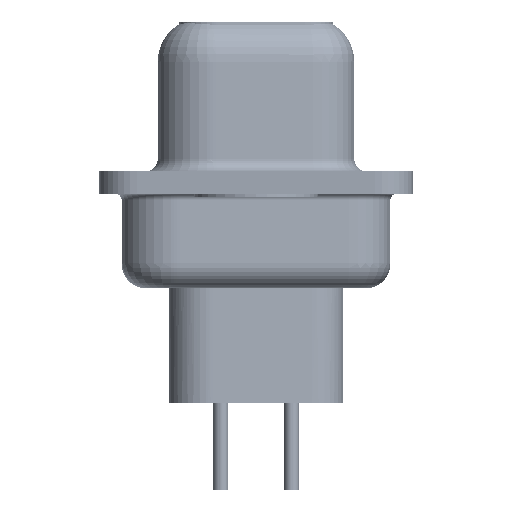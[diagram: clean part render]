
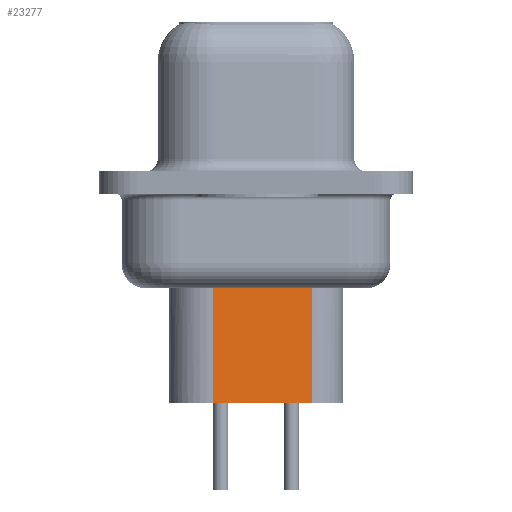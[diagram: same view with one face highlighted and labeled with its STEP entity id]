
A CAD part, left-side view. The second image highlights one B-rep face of the part: STEP entity #23277.
In plain terms, the highlighted planar face has unit normal (-0.985, -0.174, 0).
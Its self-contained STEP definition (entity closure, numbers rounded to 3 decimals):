
#81 = VERTEX_POINT ( 'NONE', #510 ) ;
#510 = CARTESIAN_POINT ( 'NONE',  ( 5.229, -2.26, -3.975 ) ) ;
#769 = EDGE_CURVE ( 'NONE', #24077, #1715, #16296, .T. ) ;
#1715 = VERTEX_POINT ( 'NONE', #2411 ) ;
#2139 = ORIENTED_EDGE ( 'NONE', *, *, #30920, .F. ) ;
#2411 = CARTESIAN_POINT ( 'NONE',  ( 4.524, 1.74, -8.85 ) ) ;
#2695 = LINE ( 'NONE', #8028, #19003 ) ;
#4652 = AXIS2_PLACEMENT_3D ( 'NONE', #15309, #24878, #22519 ) ;
#5212 = VECTOR ( 'NONE', #23368, 1000. ) ;
#5743 = PLANE ( 'NONE',  #4652 ) ;
#8028 = CARTESIAN_POINT ( 'NONE',  ( 4.353, 2.709, -3.975 ) ) ;
#12311 = CARTESIAN_POINT ( 'NONE',  ( 4.524, 1.74, -8.85 ) ) ;
#12833 = VECTOR ( 'NONE', #20156, 1000. ) ;
#12962 = LINE ( 'NONE', #22511, #12833 ) ;
#13049 = CARTESIAN_POINT ( 'NONE',  ( 4.524, 1.74, -3.975 ) ) ;
#14074 = ORIENTED_EDGE ( 'NONE', *, *, #26063, .F. ) ;
#14485 = VECTOR ( 'NONE', #24706, 1000. ) ;
#15309 = CARTESIAN_POINT ( 'NONE',  ( 4.524, 1.74, -3.1 ) ) ;
#16296 = LINE ( 'NONE', #25712, #5212 ) ;
#18550 = EDGE_CURVE ( 'NONE', #81, #24077, #2695, .T. ) ;
#19003 = VECTOR ( 'NONE', #29507, 1000. ) ;
#20156 = DIRECTION ( 'NONE',  ( 0., 0., -1. ) ) ;
#20459 = EDGE_LOOP ( 'NONE', ( #14074, #23451, #28055, #2139 ) ) ;
#22511 = CARTESIAN_POINT ( 'NONE',  ( 5.229, -2.26, -3.1 ) ) ;
#22519 = DIRECTION ( 'NONE',  ( 0.174, -0.985, 0. ) ) ;
#23277 = ADVANCED_FACE ( 'NONE', ( #24568 ), #5743, .T. ) ;
#23368 = DIRECTION ( 'NONE',  ( 0., 0., -1. ) ) ;
#23451 = ORIENTED_EDGE ( 'NONE', *, *, #18550, .T. ) ;
#24077 = VERTEX_POINT ( 'NONE', #13049 ) ;
#24449 = CARTESIAN_POINT ( 'NONE',  ( 5.229, -2.26, -8.85 ) ) ;
#24568 = FACE_OUTER_BOUND ( 'NONE', #20459, .T. ) ;
#24706 = DIRECTION ( 'NONE',  ( -0.174, 0.985, 0. ) ) ;
#24878 = DIRECTION ( 'NONE',  ( -0.985, -0.174, 0. ) ) ;
#25712 = CARTESIAN_POINT ( 'NONE',  ( 4.524, 1.74, -3.1 ) ) ;
#26063 = EDGE_CURVE ( 'NONE', #81, #28947, #12962, .T. ) ;
#26710 = LINE ( 'NONE', #12311, #14485 ) ;
#28055 = ORIENTED_EDGE ( 'NONE', *, *, #769, .T. ) ;
#28947 = VERTEX_POINT ( 'NONE', #24449 ) ;
#29507 = DIRECTION ( 'NONE',  ( -0.174, 0.985, 0. ) ) ;
#30920 = EDGE_CURVE ( 'NONE', #28947, #1715, #26710, .T. ) ;
